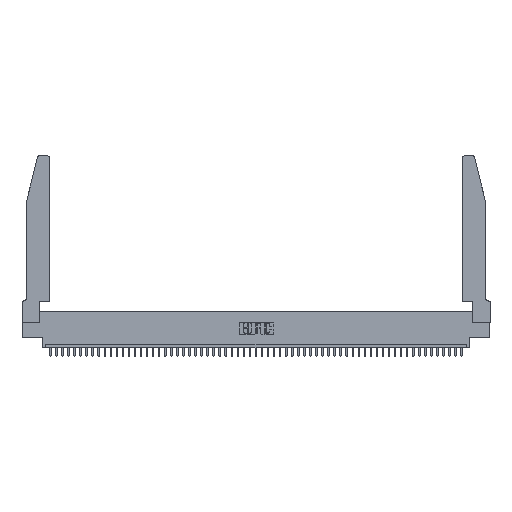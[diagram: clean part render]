
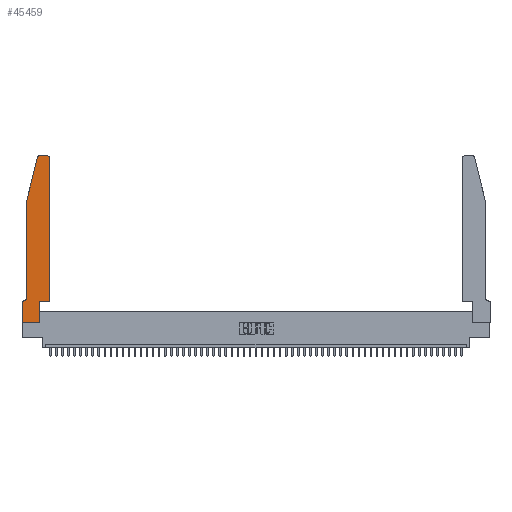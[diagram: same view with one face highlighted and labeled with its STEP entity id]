
A CAD part, top view. The second image highlights one B-rep face of the part: STEP entity #45459.
In plain terms, the highlighted planar face has unit normal (0, 0, 1).
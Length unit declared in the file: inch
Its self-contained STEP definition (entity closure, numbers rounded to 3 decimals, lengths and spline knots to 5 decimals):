
#747 = CARTESIAN_POINT ( 'NONE',  ( 0.0055, 0.35, 0.37 ) ) ;
#976 = VECTOR ( 'NONE', #15447, 39.37008 ) ;
#1418 = EDGE_CURVE ( 'NONE', #6052, #46815, #9899, .T. ) ;
#1535 = VECTOR ( 'NONE', #41628, 39.37008 ) ;
#1624 = ORIENTED_EDGE ( 'NONE', *, *, #35694, .T. ) ;
#2019 = CARTESIAN_POINT ( 'NONE',  ( 0., 0.35, 0.37 ) ) ;
#2272 = ORIENTED_EDGE ( 'NONE', *, *, #39349, .T. ) ;
#2292 = CARTESIAN_POINT ( 'NONE',  ( 0.0055, 0.42, 0.37 ) ) ;
#2890 = LINE ( 'NONE', #48353, #43946 ) ;
#3052 = DIRECTION ( 'NONE',  ( 0., 0., 1. ) ) ;
#3120 = DIRECTION ( 'NONE',  ( 0., 1., 0. ) ) ;
#3246 = DIRECTION ( 'NONE',  ( 1., 0., 0. ) ) ;
#3709 = VECTOR ( 'NONE', #47497, 39.37008 ) ;
#5742 = EDGE_CURVE ( 'NONE', #13029, #6052, #50026, .T. ) ;
#5783 = LINE ( 'NONE', #39520, #7073 ) ;
#6052 = VERTEX_POINT ( 'NONE', #32344 ) ;
#6127 = ORIENTED_EDGE ( 'NONE', *, *, #28575, .T. ) ;
#6525 = FACE_OUTER_BOUND ( 'NONE', #16227, .T. ) ;
#6682 = CARTESIAN_POINT ( 'NONE',  ( 0.0755, 2., 0.37 ) ) ;
#6753 = VECTOR ( 'NONE', #24840, 39.37008 ) ;
#6974 = CARTESIAN_POINT ( 'NONE',  ( 0.2605, 2.75, 0.37 ) ) ;
#6988 = VERTEX_POINT ( 'NONE', #20082 ) ;
#7073 = VECTOR ( 'NONE', #23000, 39.37008 ) ;
#8286 = VERTEX_POINT ( 'NONE', #25214 ) ;
#8639 = LINE ( 'NONE', #6974, #52366 ) ;
#9246 = EDGE_CURVE ( 'NONE', #46815, #6988, #13447, .T. ) ;
#9496 = DIRECTION ( 'NONE',  ( 0., 1., 0. ) ) ;
#9606 = CARTESIAN_POINT ( 'NONE',  ( 0.25487, 2.72718, 0.37 ) ) ;
#9899 = LINE ( 'NONE', #11762, #6753 ) ;
#10960 = CARTESIAN_POINT ( 'NONE',  ( 0.0755, 0.42, 0.37 ) ) ;
#10988 = CARTESIAN_POINT ( 'NONE',  ( 0.4505, 0.35, 0.37 ) ) ;
#11762 = CARTESIAN_POINT ( 'NONE',  ( 0.4505, 0.35, 0.37 ) ) ;
#13029 = VERTEX_POINT ( 'NONE', #28321 ) ;
#13447 = LINE ( 'NONE', #48894, #34586 ) ;
#13520 = ORIENTED_EDGE ( 'NONE', *, *, #9246, .T. ) ;
#14005 = DIRECTION ( 'NONE',  ( 0., 0., 1. ) ) ;
#15447 = DIRECTION ( 'NONE',  ( 0., -1., 0. ) ) ;
#15646 = AXIS2_PLACEMENT_3D ( 'NONE', #52590, #3052, #3246 ) ;
#16227 = EDGE_LOOP ( 'NONE', ( #45803, #6127, #1624, #2272, #38647, #21693, #42625, #22488, #16794, #21809, #13520, #32539 ) ) ;
#16396 = EDGE_CURVE ( 'NONE', #23787, #44841, #2890, .T. ) ;
#16521 = VERTEX_POINT ( 'NONE', #41822 ) ;
#16706 = DIRECTION ( 'NONE',  ( 0., 0., 1. ) ) ;
#16794 = ORIENTED_EDGE ( 'NONE', *, *, #5742, .T. ) ;
#17661 = VERTEX_POINT ( 'NONE', #41868 ) ;
#17759 = LINE ( 'NONE', #43315, #3709 ) ;
#18235 = CARTESIAN_POINT ( 'NONE',  ( 0.2865, 0.35, 0.37 ) ) ;
#20082 = CARTESIAN_POINT ( 'NONE',  ( 0.4505, 2.72, 0.37 ) ) ;
#21559 = EDGE_CURVE ( 'NONE', #6988, #17661, #35380, .T. ) ;
#21693 = ORIENTED_EDGE ( 'NONE', *, *, #39890, .T. ) ;
#21809 = ORIENTED_EDGE ( 'NONE', *, *, #1418, .T. ) ;
#22488 = ORIENTED_EDGE ( 'NONE', *, *, #36764, .T. ) ;
#23000 = DIRECTION ( 'NONE',  ( -0.239, -0.971, 0. ) ) ;
#23068 = DIRECTION ( 'NONE',  ( -1., 0., 0. ) ) ;
#23787 = VERTEX_POINT ( 'NONE', #28940 ) ;
#24840 = DIRECTION ( 'NONE',  ( 1., 0., 0. ) ) ;
#25214 = CARTESIAN_POINT ( 'NONE',  ( 0.0755, 2., 0.37 ) ) ;
#27466 = VERTEX_POINT ( 'NONE', #10960 ) ;
#28321 = CARTESIAN_POINT ( 'NONE',  ( 0.2865, 0., 0.37 ) ) ;
#28575 = EDGE_CURVE ( 'NONE', #16521, #32519, #42601, .T. ) ;
#28940 = CARTESIAN_POINT ( 'NONE',  ( 0., 0.35, 0.37 ) ) ;
#29397 = VECTOR ( 'NONE', #9496, 39.37008 ) ;
#29692 = LINE ( 'NONE', #50110, #1535 ) ;
#30485 = DIRECTION ( 'NONE',  ( 1., 0., 0. ) ) ;
#32344 = CARTESIAN_POINT ( 'NONE',  ( 0.2865, 0.35, 0.37 ) ) ;
#32519 = VERTEX_POINT ( 'NONE', #9606 ) ;
#32539 = ORIENTED_EDGE ( 'NONE', *, *, #21559, .T. ) ;
#34322 = AXIS2_PLACEMENT_3D ( 'NONE', #2292, #38656, #39208 ) ;
#34405 = AXIS2_PLACEMENT_3D ( 'NONE', #37142, #16706, #45455 ) ;
#34586 = VECTOR ( 'NONE', #3120, 39.37008 ) ;
#35258 = CARTESIAN_POINT ( 'NONE',  ( 0., 0., 0.37 ) ) ;
#35380 = CIRCLE ( 'NONE', #15646, 0.03 ) ;
#35694 = EDGE_CURVE ( 'NONE', #32519, #8286, #5783, .T. ) ;
#36764 = EDGE_CURVE ( 'NONE', #44841, #13029, #17759, .T. ) ;
#37142 = CARTESIAN_POINT ( 'NONE',  ( 0.284, 2.72, 0.37 ) ) ;
#38141 = EDGE_CURVE ( 'NONE', #17661, #16521, #8639, .T. ) ;
#38647 = ORIENTED_EDGE ( 'NONE', *, *, #48473, .T. ) ;
#38656 = DIRECTION ( 'NONE',  ( 0., 0., -1. ) ) ;
#39208 = DIRECTION ( 'NONE',  ( -1., 0., 0. ) ) ;
#39349 = EDGE_CURVE ( 'NONE', #8286, #27466, #53024, .T. ) ;
#39520 = CARTESIAN_POINT ( 'NONE',  ( 0.0755, 2., 0.37 ) ) ;
#39612 = VERTEX_POINT ( 'NONE', #747 ) ;
#39890 = EDGE_CURVE ( 'NONE', #39612, #23787, #29692, .T. ) ;
#41628 = DIRECTION ( 'NONE',  ( -1., 0., 0. ) ) ;
#41822 = CARTESIAN_POINT ( 'NONE',  ( 0.284, 2.75, 0.37 ) ) ;
#41868 = CARTESIAN_POINT ( 'NONE',  ( 0.4205, 2.75, 0.37 ) ) ;
#42601 = CIRCLE ( 'NONE', #34405, 0.03 ) ;
#42625 = ORIENTED_EDGE ( 'NONE', *, *, #16396, .T. ) ;
#42681 = CIRCLE ( 'NONE', #34322, 0.07 ) ;
#43078 = PLANE ( 'NONE',  #44604 ) ;
#43315 = CARTESIAN_POINT ( 'NONE',  ( 0., 0., 0.37 ) ) ;
#43946 = VECTOR ( 'NONE', #44360, 39.37008 ) ;
#44360 = DIRECTION ( 'NONE',  ( 0., -1., 0. ) ) ;
#44604 = AXIS2_PLACEMENT_3D ( 'NONE', #2019, #14005, #30485 ) ;
#44841 = VERTEX_POINT ( 'NONE', #35258 ) ;
#45455 = DIRECTION ( 'NONE',  ( 1., 0., 0. ) ) ;
#45459 = ADVANCED_FACE ( 'NONE', ( #6525 ), #43078, .T. ) ;
#45803 = ORIENTED_EDGE ( 'NONE', *, *, #38141, .T. ) ;
#46815 = VERTEX_POINT ( 'NONE', #10988 ) ;
#47497 = DIRECTION ( 'NONE',  ( 1., 0., 0. ) ) ;
#48353 = CARTESIAN_POINT ( 'NONE',  ( 0., 0., 0.37 ) ) ;
#48473 = EDGE_CURVE ( 'NONE', #27466, #39612, #42681, .T. ) ;
#48894 = CARTESIAN_POINT ( 'NONE',  ( 0.4505, 0.35, 0.37 ) ) ;
#50026 = LINE ( 'NONE', #18235, #29397 ) ;
#50110 = CARTESIAN_POINT ( 'NONE',  ( 0.0755, 0.35, 0.37 ) ) ;
#52366 = VECTOR ( 'NONE', #23068, 39.37008 ) ;
#52590 = CARTESIAN_POINT ( 'NONE',  ( 0.4205, 2.72, 0.37 ) ) ;
#53024 = LINE ( 'NONE', #6682, #976 ) ;
